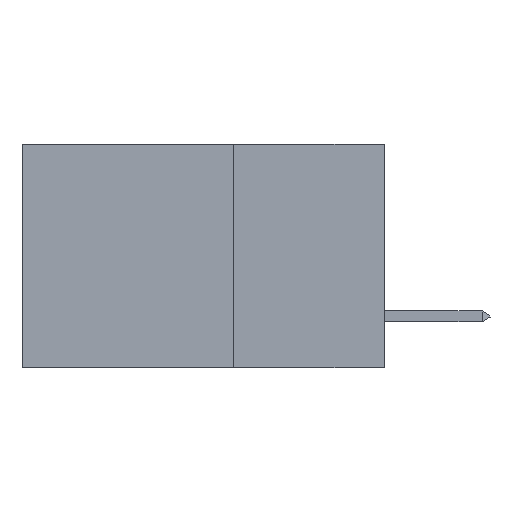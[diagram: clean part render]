
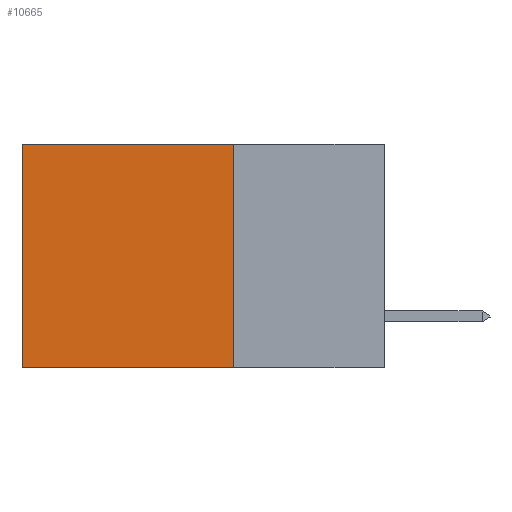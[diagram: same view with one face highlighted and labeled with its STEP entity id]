
A CAD part, left-side view. The second image highlights one B-rep face of the part: STEP entity #10665.
In plain terms, the highlighted planar face has unit normal (-1, 0, 0).
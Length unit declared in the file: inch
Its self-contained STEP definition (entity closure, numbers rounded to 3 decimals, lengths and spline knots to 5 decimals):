
#361 = ORIENTED_EDGE ( 'NONE', *, *, #31169, .T. ) ;
#712 = CARTESIAN_POINT ( 'NONE',  ( 0.2875, 0.25, 0. ) ) ;
#1980 = EDGE_CURVE ( 'NONE', #19376, #3200, #6252, .T. ) ;
#3200 = VERTEX_POINT ( 'NONE', #23186 ) ;
#4082 = DIRECTION ( 'NONE',  ( 0., 0., -1. ) ) ;
#5031 = DIRECTION ( 'NONE',  ( 0., 0., -1. ) ) ;
#6252 = LINE ( 'NONE', #6591, #18346 ) ;
#6591 = CARTESIAN_POINT ( 'NONE',  ( 0.2875, 0.25, -0.37 ) ) ;
#7410 = CARTESIAN_POINT ( 'NONE',  ( 0.2875, 0.6, 0. ) ) ;
#7973 = DIRECTION ( 'NONE',  ( 0., 1., 0. ) ) ;
#8805 = CARTESIAN_POINT ( 'NONE',  ( 0.2875, 0.25, 0. ) ) ;
#10157 = VERTEX_POINT ( 'NONE', #19777 ) ;
#10665 = ADVANCED_FACE ( 'NONE', ( #32153 ), #16423, .F. ) ;
#11506 = ORIENTED_EDGE ( 'NONE', *, *, #1980, .F. ) ;
#12156 = VECTOR ( 'NONE', #5031, 39.37008 ) ;
#16423 = PLANE ( 'NONE',  #18600 ) ;
#16636 = CARTESIAN_POINT ( 'NONE',  ( 0.2875, 0.25, -0.37 ) ) ;
#17467 = ORIENTED_EDGE ( 'NONE', *, *, #20956, .T. ) ;
#18346 = VECTOR ( 'NONE', #21656, 39.37008 ) ;
#18412 = LINE ( 'NONE', #30015, #12156 ) ;
#18426 = EDGE_LOOP ( 'NONE', ( #361, #11506, #24204, #17467 ) ) ;
#18600 = AXIS2_PLACEMENT_3D ( 'NONE', #8805, #31482, #4082 ) ;
#19061 = LINE ( 'NONE', #7410, #21757 ) ;
#19376 = VERTEX_POINT ( 'NONE', #16636 ) ;
#19507 = CARTESIAN_POINT ( 'NONE',  ( 0.2875, 0.25, 0. ) ) ;
#19777 = CARTESIAN_POINT ( 'NONE',  ( 0.2875, 0.6, 0. ) ) ;
#20254 = VECTOR ( 'NONE', #7973, 39.37008 ) ;
#20956 = EDGE_CURVE ( 'NONE', #27105, #10157, #31216, .T. ) ;
#21656 = DIRECTION ( 'NONE',  ( 0., 1., 0. ) ) ;
#21757 = VECTOR ( 'NONE', #29876, 39.37008 ) ;
#23186 = CARTESIAN_POINT ( 'NONE',  ( 0.2875, 0.6, -0.37 ) ) ;
#24204 = ORIENTED_EDGE ( 'NONE', *, *, #29056, .F. ) ;
#27105 = VERTEX_POINT ( 'NONE', #19507 ) ;
#29056 = EDGE_CURVE ( 'NONE', #27105, #19376, #18412, .T. ) ;
#29876 = DIRECTION ( 'NONE',  ( 0., 0., -1. ) ) ;
#30015 = CARTESIAN_POINT ( 'NONE',  ( 0.2875, 0.25, 0. ) ) ;
#31169 = EDGE_CURVE ( 'NONE', #10157, #3200, #19061, .T. ) ;
#31216 = LINE ( 'NONE', #712, #20254 ) ;
#31482 = DIRECTION ( 'NONE',  ( 1., 0., 0. ) ) ;
#32153 = FACE_OUTER_BOUND ( 'NONE', #18426, .T. ) ;
